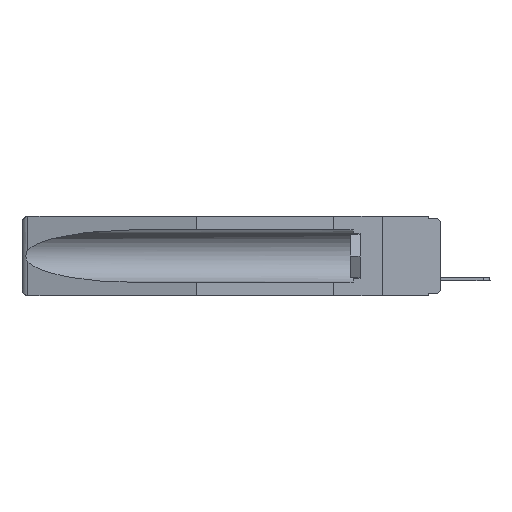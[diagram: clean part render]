
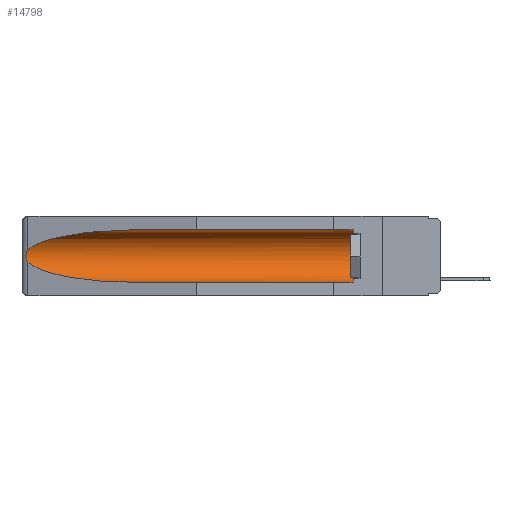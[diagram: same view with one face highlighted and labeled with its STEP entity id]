
A CAD part, left-side view. The second image highlights one B-rep face of the part: STEP entity #14798.
In plain terms, the highlighted cylindrical face has radius 2.857 mm (diameter 5.715 mm), a partial arc.
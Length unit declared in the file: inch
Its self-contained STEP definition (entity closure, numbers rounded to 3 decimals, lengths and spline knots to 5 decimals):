
#207 = ORIENTED_EDGE ( 'NONE', *, *, #8960, .T. ) ;
#484 = CARTESIAN_POINT ( 'NONE',  ( 0.155, 0.126, -0.284 ) ) ;
#678 = LINE ( 'NONE', #14523, #17734 ) ;
#1027 = CARTESIAN_POINT ( 'NONE',  ( 0.155, 1.07973, -0.284 ) ) ;
#1131 =( BOUNDED_CURVE ( )  B_SPLINE_CURVE ( 3, ( #16522, #8992, #9191, #1027 ),
 .UNSPECIFIED., .F., .F. ) 
 B_SPLINE_CURVE_WITH_KNOTS ( ( 4, 4 ),
 ( 0.1948, 1.5708 ),
 .UNSPECIFIED. ) 
 CURVE ( )  GEOMETRIC_REPRESENTATION_ITEM ( )  RATIONAL_B_SPLINE_CURVE ( ( 1., 0.848, 0.848, 1. ) ) 
 REPRESENTATION_ITEM ( '' )  );
#1551 = VERTEX_POINT ( 'NONE', #12950 ) ;
#1628 = DIRECTION ( 'NONE',  ( 0., 0., 1. ) ) ;
#1629 = CARTESIAN_POINT ( 'NONE',  ( 0.155, -0.30754, -0.1715 ) ) ;
#1940 = B_SPLINE_CURVE_WITH_KNOTS ( 'NONE', 3,
 ( #19325, #4755, #12487, #6200, #7830, #3229, #12981, #2091, #14012, #8411 ),
 .UNSPECIFIED., .F., .F.,
 ( 4, 2, 2, 2, 4 ),
 ( 0., 0.00029, 0.00058, 0.00087, 0.00117 ),
 .UNSPECIFIED. ) ;
#2091 = CARTESIAN_POINT ( 'NONE',  ( 0.26655, 1.53094, -0.18657 ) ) ;
#2180 = LINE ( 'NONE', #11540, #15305 ) ;
#2291 = ORIENTED_EDGE ( 'NONE', *, *, #12855, .T. ) ;
#3214 = ORIENTED_EDGE ( 'NONE', *, *, #16583, .T. ) ;
#3229 = CARTESIAN_POINT ( 'NONE',  ( 0.2675, 1.53308, -0.17534 ) ) ;
#3293 = EDGE_CURVE ( 'NONE', #1551, #19308, #13628, .T. ) ;
#4026 = CARTESIAN_POINT ( 'NONE',  ( 0.26537, 1.52718, -0.14972 ) ) ;
#4264 = CARTESIAN_POINT ( 'NONE',  ( 0.25451, 1.48313, -0.09465 ) ) ;
#4361 = CARTESIAN_POINT ( 'NONE',  ( 0.26537, 1.52718, -0.14972 ) ) ;
#4755 = CARTESIAN_POINT ( 'NONE',  ( 0.26597, 1.52961, -0.15275 ) ) ;
#4924 = ORIENTED_EDGE ( 'NONE', *, *, #12714, .F. ) ;
#4967 = ORIENTED_EDGE ( 'NONE', *, *, #3293, .T. ) ;
#5384 = AXIS2_PLACEMENT_3D ( 'NONE', #1629, #13742, #13839 ) ;
#6042 = ORIENTED_EDGE ( 'NONE', *, *, #6384, .T. ) ;
#6200 = CARTESIAN_POINT ( 'NONE',  ( 0.2673, 1.5327, -0.16383 ) ) ;
#6384 = EDGE_CURVE ( 'NONE', #8129, #15357, #16255, .T. ) ;
#6522 = AXIS2_PLACEMENT_3D ( 'NONE', #11113, #10900, #1628 ) ;
#7529 = CARTESIAN_POINT ( 'NONE',  ( 0.26537, 1.52718, -0.19328 ) ) ;
#7830 = CARTESIAN_POINT ( 'NONE',  ( 0.2675, 1.53308, -0.16763 ) ) ;
#8129 = VERTEX_POINT ( 'NONE', #484 ) ;
#8411 = CARTESIAN_POINT ( 'NONE',  ( 0.26537, 1.52718, -0.19328 ) ) ;
#8960 = EDGE_CURVE ( 'NONE', #15357, #1551, #2180, .T. ) ;
#8964 = CARTESIAN_POINT ( 'NONE',  ( 0.155, 0.126, -0.059 ) ) ;
#8992 = CARTESIAN_POINT ( 'NONE',  ( 0.25451, 1.48313, -0.24835 ) ) ;
#9191 = CARTESIAN_POINT ( 'NONE',  ( 0.21114, 1.30732, -0.284 ) ) ;
#9616 = VERTEX_POINT ( 'NONE', #7529 ) ;
#10013 = CARTESIAN_POINT ( 'NONE',  ( 0.155, 1.07973, -0.284 ) ) ;
#10900 = DIRECTION ( 'NONE',  ( 0., -1., 0. ) ) ;
#11005 = FACE_OUTER_BOUND ( 'NONE', #17934, .T. ) ;
#11113 = CARTESIAN_POINT ( 'NONE',  ( 0.155, 0.126, -0.1715 ) ) ;
#11540 = CARTESIAN_POINT ( 'NONE',  ( 0.155, -0.30754, -0.059 ) ) ;
#12487 = CARTESIAN_POINT ( 'NONE',  ( 0.26654, 1.53092, -0.15636 ) ) ;
#12714 = EDGE_CURVE ( 'NONE', #8129, #13473, #678, .T. ) ;
#12855 = EDGE_CURVE ( 'NONE', #19308, #9616, #1940, .T. ) ;
#12950 = CARTESIAN_POINT ( 'NONE',  ( 0.155, 1.07973, -0.059 ) ) ;
#12981 = CARTESIAN_POINT ( 'NONE',  ( 0.2673, 1.53269, -0.17917 ) ) ;
#13009 = DIRECTION ( 'NONE',  ( 0., 1., 0. ) ) ;
#13473 = VERTEX_POINT ( 'NONE', #10013 ) ;
#13623 = CARTESIAN_POINT ( 'NONE',  ( 0.155, 1.07973, -0.059 ) ) ;
#13628 =( BOUNDED_CURVE ( )  B_SPLINE_CURVE ( 3, ( #13623, #18242, #4264, #4361 ),
 .UNSPECIFIED., .F., .F. ) 
 B_SPLINE_CURVE_WITH_KNOTS ( ( 4, 4 ),
 ( 4.71239, 6.08839 ),
 .UNSPECIFIED. ) 
 CURVE ( )  GEOMETRIC_REPRESENTATION_ITEM ( )  RATIONAL_B_SPLINE_CURVE ( ( 1., 0.848, 0.848, 1. ) ) 
 REPRESENTATION_ITEM ( '' )  );
#13742 = DIRECTION ( 'NONE',  ( 0., 1., 0. ) ) ;
#13839 = DIRECTION ( 'NONE',  ( 0., 0., 1. ) ) ;
#14012 = CARTESIAN_POINT ( 'NONE',  ( 0.26597, 1.5296, -0.19026 ) ) ;
#14523 = CARTESIAN_POINT ( 'NONE',  ( 0.155, -0.30754, -0.284 ) ) ;
#14798 = ADVANCED_FACE ( 'NONE', ( #11005 ), #14999, .F. ) ;
#14999 = CYLINDRICAL_SURFACE ( 'NONE', #5384, 0.1125 ) ;
#15305 = VECTOR ( 'NONE', #17768, 39.37008 ) ;
#15357 = VERTEX_POINT ( 'NONE', #8964 ) ;
#16255 = CIRCLE ( 'NONE', #6522, 0.1125 ) ;
#16522 = CARTESIAN_POINT ( 'NONE',  ( 0.26537, 1.52718, -0.19328 ) ) ;
#16583 = EDGE_CURVE ( 'NONE', #9616, #13473, #1131, .T. ) ;
#17734 = VECTOR ( 'NONE', #13009, 39.37008 ) ;
#17768 = DIRECTION ( 'NONE',  ( 0., 1., 0. ) ) ;
#17934 = EDGE_LOOP ( 'NONE', ( #4967, #2291, #3214, #4924, #6042, #207 ) ) ;
#18242 = CARTESIAN_POINT ( 'NONE',  ( 0.21114, 1.30732, -0.059 ) ) ;
#19308 = VERTEX_POINT ( 'NONE', #4026 ) ;
#19325 = CARTESIAN_POINT ( 'NONE',  ( 0.26537, 1.52718, -0.14972 ) ) ;
